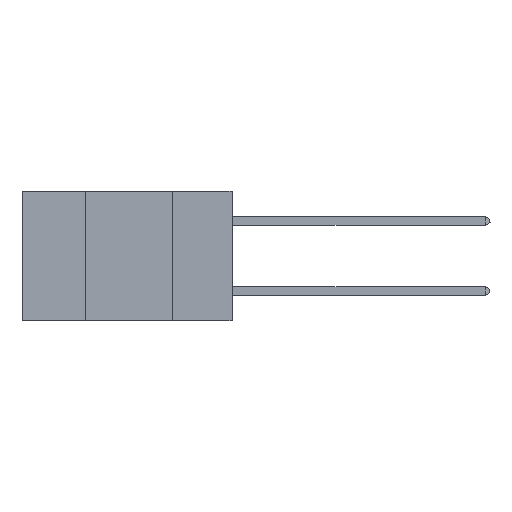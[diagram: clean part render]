
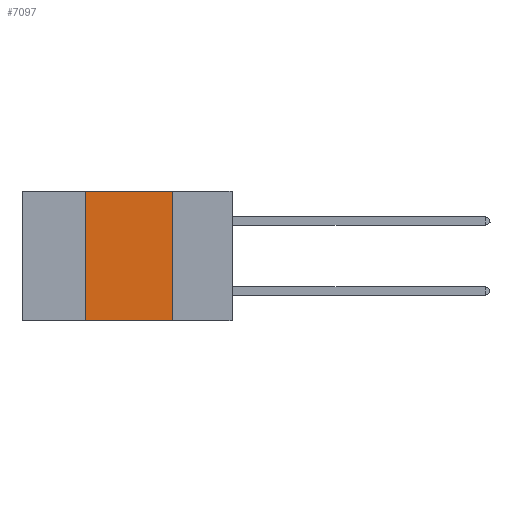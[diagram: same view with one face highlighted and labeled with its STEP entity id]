
A CAD part, left-side view. The second image highlights one B-rep face of the part: STEP entity #7097.
In plain terms, the highlighted planar face has unit normal (-1, 0, 0).
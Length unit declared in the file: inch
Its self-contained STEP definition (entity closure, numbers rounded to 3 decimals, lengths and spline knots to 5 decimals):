
#1743 = CARTESIAN_POINT ( 'NONE',  ( 0., 0.17, 0. ) ) ;
#2607 = FACE_OUTER_BOUND ( 'NONE', #5424, .T. ) ;
#3264 = VECTOR ( 'NONE', #38016, 39.37008 ) ;
#3309 = CARTESIAN_POINT ( 'NONE',  ( 0., 0.6, 0. ) ) ;
#5109 = CARTESIAN_POINT ( 'NONE',  ( 0., 0.6, 0. ) ) ;
#5424 = EDGE_LOOP ( 'NONE', ( #19852, #39653, #44791, #45326 ) ) ;
#7097 = ADVANCED_FACE ( 'NONE', ( #2607 ), #39741, .F. ) ;
#9183 = LINE ( 'NONE', #28525, #47327 ) ;
#9414 = CARTESIAN_POINT ( 'NONE',  ( 0., 0.42, 0. ) ) ;
#11451 = CARTESIAN_POINT ( 'NONE',  ( 0., 0.42, -0.37 ) ) ;
#14560 = VECTOR ( 'NONE', #19451, 39.37008 ) ;
#19221 = LINE ( 'NONE', #41538, #14560 ) ;
#19451 = DIRECTION ( 'NONE',  ( 0., -1., 0. ) ) ;
#19706 = VERTEX_POINT ( 'NONE', #9414 ) ;
#19852 = ORIENTED_EDGE ( 'NONE', *, *, #36183, .F. ) ;
#19942 = DIRECTION ( 'NONE',  ( 0., -1., 0. ) ) ;
#21168 = VERTEX_POINT ( 'NONE', #11451 ) ;
#24723 = DIRECTION ( 'NONE',  ( 0., 0., -1. ) ) ;
#24933 = VECTOR ( 'NONE', #19942, 39.37008 ) ;
#28525 = CARTESIAN_POINT ( 'NONE',  ( 0., 0.42, 0. ) ) ;
#29734 = AXIS2_PLACEMENT_3D ( 'NONE', #3309, #43654, #24723 ) ;
#30663 = CARTESIAN_POINT ( 'NONE',  ( 0., 0.17, 0. ) ) ;
#31204 = VERTEX_POINT ( 'NONE', #41917 ) ;
#33635 = EDGE_CURVE ( 'NONE', #21168, #31204, #19221, .T. ) ;
#34343 = VERTEX_POINT ( 'NONE', #30663 ) ;
#35611 = DIRECTION ( 'NONE',  ( 0., 0., 1. ) ) ;
#36183 = EDGE_CURVE ( 'NONE', #34343, #31204, #42505, .T. ) ;
#38016 = DIRECTION ( 'NONE',  ( 0., 0., -1. ) ) ;
#39653 = ORIENTED_EDGE ( 'NONE', *, *, #40861, .F. ) ;
#39741 = PLANE ( 'NONE',  #29734 ) ;
#40861 = EDGE_CURVE ( 'NONE', #19706, #34343, #41170, .T. ) ;
#41170 = LINE ( 'NONE', #5109, #24933 ) ;
#41538 = CARTESIAN_POINT ( 'NONE',  ( 0., 0.6, -0.37 ) ) ;
#41917 = CARTESIAN_POINT ( 'NONE',  ( 0., 0.17, -0.37 ) ) ;
#42505 = LINE ( 'NONE', #1743, #3264 ) ;
#43654 = DIRECTION ( 'NONE',  ( 1., 0., 0. ) ) ;
#44791 = ORIENTED_EDGE ( 'NONE', *, *, #47866, .F. ) ;
#45326 = ORIENTED_EDGE ( 'NONE', *, *, #33635, .T. ) ;
#47327 = VECTOR ( 'NONE', #35611, 39.37008 ) ;
#47866 = EDGE_CURVE ( 'NONE', #21168, #19706, #9183, .T. ) ;
